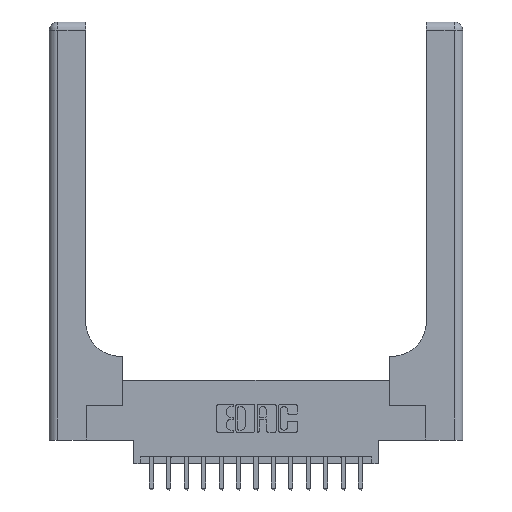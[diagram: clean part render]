
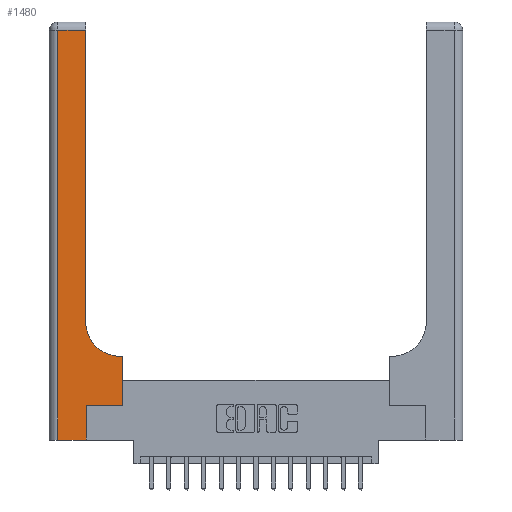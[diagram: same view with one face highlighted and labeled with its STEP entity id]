
A CAD part, top view. The second image highlights one B-rep face of the part: STEP entity #1480.
In plain terms, the highlighted planar face has unit normal (0, 0, 1).
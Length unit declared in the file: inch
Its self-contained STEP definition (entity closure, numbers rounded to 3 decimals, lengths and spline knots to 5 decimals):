
#117 = ORIENTED_EDGE ( 'NONE', *, *, #15264, .T. ) ;
#141 = FACE_OUTER_BOUND ( 'NONE', #8052, .T. ) ;
#354 = VECTOR ( 'NONE', #5351, 39.37008 ) ;
#422 = DIRECTION ( 'NONE',  ( -1., 0., 0. ) ) ;
#482 = EDGE_CURVE ( 'NONE', #12665, #17496, #4529, .T. ) ;
#936 = LINE ( 'NONE', #9620, #354 ) ;
#1061 = CARTESIAN_POINT ( 'NONE',  ( 0.528, 0.25, 0.37 ) ) ;
#1135 = VECTOR ( 'NONE', #12542, 39.37008 ) ;
#1439 = CARTESIAN_POINT ( 'NONE',  ( 0.528, 0.6, 0.37 ) ) ;
#1480 = ADVANCED_FACE ( 'NONE', ( #141 ), #14466, .F. ) ;
#1810 = LINE ( 'NONE', #15841, #11476 ) ;
#1840 = CARTESIAN_POINT ( 'NONE',  ( 0., 2.94, 0.37 ) ) ;
#2135 = CARTESIAN_POINT ( 'NONE',  ( 0.26, 0.85, 0.37 ) ) ;
#2361 = CARTESIAN_POINT ( 'NONE',  ( 0.528, 0.25, 0.37 ) ) ;
#3562 = EDGE_CURVE ( 'NONE', #14893, #10843, #8743, .T. ) ;
#3980 = EDGE_CURVE ( 'NONE', #17496, #5310, #14001, .T. ) ;
#4289 = CARTESIAN_POINT ( 'NONE',  ( 0., 3., 0.37 ) ) ;
#4529 = LINE ( 'NONE', #10180, #5250 ) ;
#4616 = DIRECTION ( 'NONE',  ( 1., 0., 0. ) ) ;
#5250 = VECTOR ( 'NONE', #4616, 39.37008 ) ;
#5310 = VERTEX_POINT ( 'NONE', #1439 ) ;
#5351 = DIRECTION ( 'NONE',  ( 0., -1., 0. ) ) ;
#6056 = DIRECTION ( 'NONE',  ( 0., 1., 0. ) ) ;
#6120 = VECTOR ( 'NONE', #11977, 39.37008 ) ;
#6283 = EDGE_CURVE ( 'NONE', #14366, #14893, #14940, .T. ) ;
#6426 = CARTESIAN_POINT ( 'NONE',  ( 0.06, 2.94, 0.37 ) ) ;
#7476 = LINE ( 'NONE', #1840, #12701 ) ;
#7715 = VERTEX_POINT ( 'NONE', #13308 ) ;
#7939 = CARTESIAN_POINT ( 'NONE',  ( 0., 0., 0.37 ) ) ;
#7994 = DIRECTION ( 'NONE',  ( 0., 1., 0. ) ) ;
#8052 = EDGE_LOOP ( 'NONE', ( #11715, #117, #17902, #8335, #13877, #11915, #15053, #15172, #14716 ) ) ;
#8335 = ORIENTED_EDGE ( 'NONE', *, *, #9334, .T. ) ;
#8743 = LINE ( 'NONE', #10116, #15746 ) ;
#9101 = CARTESIAN_POINT ( 'NONE',  ( 0.06, 0., 0.37 ) ) ;
#9330 = LINE ( 'NONE', #7939, #6120 ) ;
#9334 = EDGE_CURVE ( 'NONE', #16248, #7715, #9330, .T. ) ;
#9354 = AXIS2_PLACEMENT_3D ( 'NONE', #13025, #14247, #11721 ) ;
#9530 = CARTESIAN_POINT ( 'NONE',  ( 0.265, 0.25, 0.37 ) ) ;
#9620 = CARTESIAN_POINT ( 'NONE',  ( 0.06, 3., 0.37 ) ) ;
#9865 = CARTESIAN_POINT ( 'NONE',  ( 0.51, 0.6, 0.37 ) ) ;
#10116 = CARTESIAN_POINT ( 'NONE',  ( 0.26, 3., 0.37 ) ) ;
#10180 = CARTESIAN_POINT ( 'NONE',  ( 0.265, 0.25, 0.37 ) ) ;
#10481 = EDGE_CURVE ( 'NONE', #5310, #14366, #13860, .T. ) ;
#10843 = VERTEX_POINT ( 'NONE', #17709 ) ;
#11329 = AXIS2_PLACEMENT_3D ( 'NONE', #4289, #15934, #422 ) ;
#11476 = VECTOR ( 'NONE', #6056, 39.37008 ) ;
#11715 = ORIENTED_EDGE ( 'NONE', *, *, #3562, .T. ) ;
#11721 = DIRECTION ( 'NONE',  ( 1., 0., 0. ) ) ;
#11904 = VECTOR ( 'NONE', #7994, 39.37008 ) ;
#11915 = ORIENTED_EDGE ( 'NONE', *, *, #482, .T. ) ;
#11977 = DIRECTION ( 'NONE',  ( 1., 0., 0. ) ) ;
#12213 = EDGE_CURVE ( 'NONE', #7715, #12665, #1810, .T. ) ;
#12542 = DIRECTION ( 'NONE',  ( -1., 0., 0. ) ) ;
#12665 = VERTEX_POINT ( 'NONE', #9530 ) ;
#12701 = VECTOR ( 'NONE', #17258, 39.37008 ) ;
#13025 = CARTESIAN_POINT ( 'NONE',  ( 0.51, 0.85, 0.37 ) ) ;
#13308 = CARTESIAN_POINT ( 'NONE',  ( 0.265, 0., 0.37 ) ) ;
#13860 = LINE ( 'NONE', #15327, #1135 ) ;
#13877 = ORIENTED_EDGE ( 'NONE', *, *, #12213, .T. ) ;
#14001 = LINE ( 'NONE', #2361, #11904 ) ;
#14247 = DIRECTION ( 'NONE',  ( 0., 0., -1. ) ) ;
#14366 = VERTEX_POINT ( 'NONE', #9865 ) ;
#14377 = DIRECTION ( 'NONE',  ( 0., 1., 0. ) ) ;
#14466 = PLANE ( 'NONE',  #11329 ) ;
#14597 = VERTEX_POINT ( 'NONE', #6426 ) ;
#14716 = ORIENTED_EDGE ( 'NONE', *, *, #6283, .T. ) ;
#14893 = VERTEX_POINT ( 'NONE', #2135 ) ;
#14940 = CIRCLE ( 'NONE', #9354, 0.25 ) ;
#14964 = EDGE_CURVE ( 'NONE', #14597, #16248, #936, .T. ) ;
#15053 = ORIENTED_EDGE ( 'NONE', *, *, #3980, .T. ) ;
#15172 = ORIENTED_EDGE ( 'NONE', *, *, #10481, .T. ) ;
#15264 = EDGE_CURVE ( 'NONE', #10843, #14597, #7476, .T. ) ;
#15327 = CARTESIAN_POINT ( 'NONE',  ( 0.26, 0.6, 0.37 ) ) ;
#15746 = VECTOR ( 'NONE', #14377, 39.37008 ) ;
#15841 = CARTESIAN_POINT ( 'NONE',  ( 0.265, 0., 0.37 ) ) ;
#15934 = DIRECTION ( 'NONE',  ( 0., 0., -1. ) ) ;
#16248 = VERTEX_POINT ( 'NONE', #9101 ) ;
#17258 = DIRECTION ( 'NONE',  ( -1., 0., 0. ) ) ;
#17496 = VERTEX_POINT ( 'NONE', #1061 ) ;
#17709 = CARTESIAN_POINT ( 'NONE',  ( 0.26, 2.94, 0.37 ) ) ;
#17902 = ORIENTED_EDGE ( 'NONE', *, *, #14964, .T. ) ;
